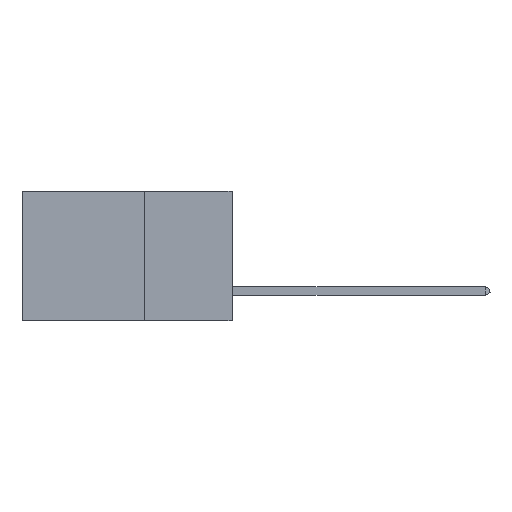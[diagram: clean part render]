
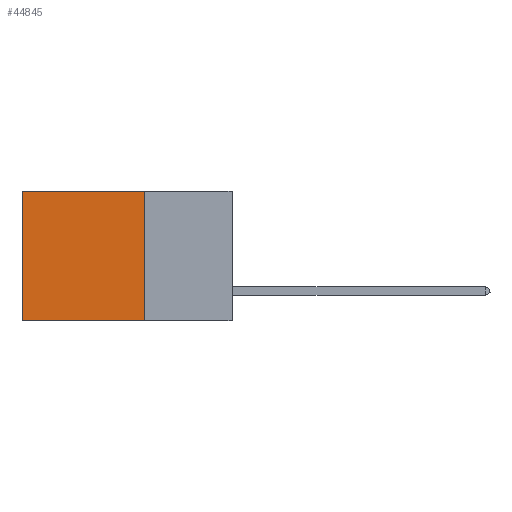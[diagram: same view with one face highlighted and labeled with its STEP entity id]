
A CAD part, left-side view. The second image highlights one B-rep face of the part: STEP entity #44845.
In plain terms, the highlighted planar face has unit normal (-1, 0, 0).
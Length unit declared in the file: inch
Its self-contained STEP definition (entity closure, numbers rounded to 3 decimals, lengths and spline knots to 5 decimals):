
#162 = DIRECTION ( 'NONE',  ( 0., 0., -1. ) ) ;
#323 = EDGE_CURVE ( 'NONE', #13018, #38494, #5346, .T. ) ;
#1441 = PLANE ( 'NONE',  #22860 ) ;
#2716 = VERTEX_POINT ( 'NONE', #2937 ) ;
#2937 = CARTESIAN_POINT ( 'NONE',  ( 0.2875, 0.25, -0.37 ) ) ;
#5346 = LINE ( 'NONE', #40490, #35825 ) ;
#6100 = DIRECTION ( 'NONE',  ( 0., 0., -1. ) ) ;
#6610 = ORIENTED_EDGE ( 'NONE', *, *, #323, .T. ) ;
#7894 = DIRECTION ( 'NONE',  ( 0., 1., 0. ) ) ;
#8950 = VECTOR ( 'NONE', #7894, 39.37008 ) ;
#9687 = ORIENTED_EDGE ( 'NONE', *, *, #21960, .T. ) ;
#11379 = CARTESIAN_POINT ( 'NONE',  ( 0.2875, 0.25, 0. ) ) ;
#11511 = ORIENTED_EDGE ( 'NONE', *, *, #33743, .F. ) ;
#11784 = LINE ( 'NONE', #33225, #38920 ) ;
#13018 = VERTEX_POINT ( 'NONE', #14760 ) ;
#13692 = VECTOR ( 'NONE', #13992, 39.37008 ) ;
#13821 = EDGE_LOOP ( 'NONE', ( #6610, #15607, #11511, #9687 ) ) ;
#13992 = DIRECTION ( 'NONE',  ( 0., 1., 0. ) ) ;
#14760 = CARTESIAN_POINT ( 'NONE',  ( 0.2875, 0.6, 0. ) ) ;
#15607 = ORIENTED_EDGE ( 'NONE', *, *, #17130, .F. ) ;
#16232 = DIRECTION ( 'NONE',  ( 1., 0., 0. ) ) ;
#17130 = EDGE_CURVE ( 'NONE', #2716, #38494, #37154, .T. ) ;
#17693 = CARTESIAN_POINT ( 'NONE',  ( 0.2875, 0.25, 0. ) ) ;
#21960 = EDGE_CURVE ( 'NONE', #36312, #13018, #44741, .T. ) ;
#22064 = CARTESIAN_POINT ( 'NONE',  ( 0.2875, 0.6, -0.37 ) ) ;
#22860 = AXIS2_PLACEMENT_3D ( 'NONE', #30899, #16232, #6100 ) ;
#30899 = CARTESIAN_POINT ( 'NONE',  ( 0.2875, 0.25, 0. ) ) ;
#33225 = CARTESIAN_POINT ( 'NONE',  ( 0.2875, 0.25, 0. ) ) ;
#33743 = EDGE_CURVE ( 'NONE', #36312, #2716, #11784, .T. ) ;
#35825 = VECTOR ( 'NONE', #162, 39.37008 ) ;
#36312 = VERTEX_POINT ( 'NONE', #11379 ) ;
#36483 = FACE_OUTER_BOUND ( 'NONE', #13821, .T. ) ;
#37154 = LINE ( 'NONE', #46758, #8950 ) ;
#38494 = VERTEX_POINT ( 'NONE', #22064 ) ;
#38920 = VECTOR ( 'NONE', #40593, 39.37008 ) ;
#40490 = CARTESIAN_POINT ( 'NONE',  ( 0.2875, 0.6, 0. ) ) ;
#40593 = DIRECTION ( 'NONE',  ( 0., 0., -1. ) ) ;
#44741 = LINE ( 'NONE', #17693, #13692 ) ;
#44845 = ADVANCED_FACE ( 'NONE', ( #36483 ), #1441, .F. ) ;
#46758 = CARTESIAN_POINT ( 'NONE',  ( 0.2875, 0.25, -0.37 ) ) ;
